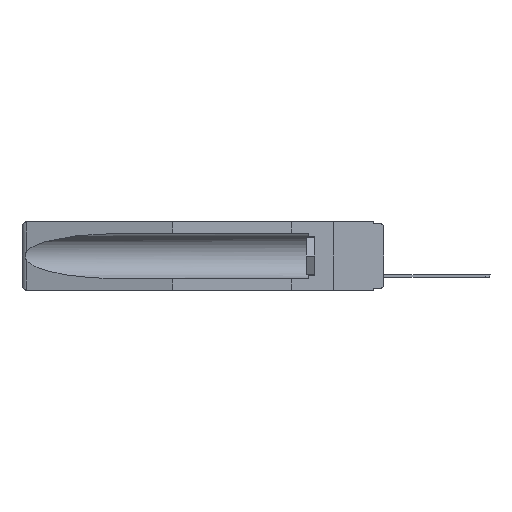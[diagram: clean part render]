
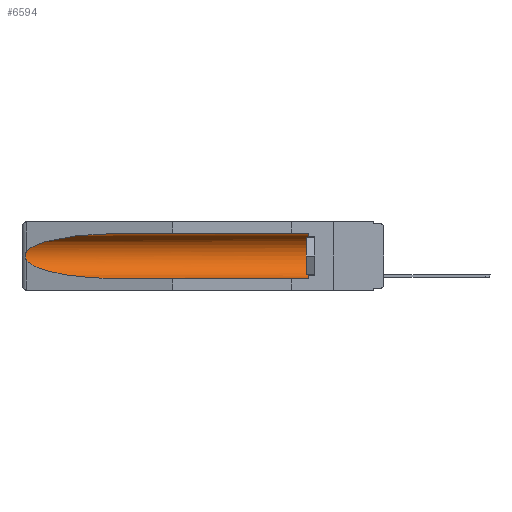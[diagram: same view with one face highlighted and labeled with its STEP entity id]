
A CAD part, left-side view. The second image highlights one B-rep face of the part: STEP entity #6594.
In plain terms, the highlighted cylindrical face has radius 2.857 mm (diameter 5.715 mm), a partial arc.
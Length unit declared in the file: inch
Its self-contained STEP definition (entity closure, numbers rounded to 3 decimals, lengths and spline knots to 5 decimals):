
#85 = VERTEX_POINT ( 'NONE', #4354 ) ;
#1199 = B_SPLINE_CURVE_WITH_KNOTS ( 'NONE', 3,
 ( #7776, #9515, #6013, #18506, #2538, #16663, #20144, #16814, #13372, #14959 ),
 .UNSPECIFIED., .F., .F.,
 ( 4, 2, 2, 2, 4 ),
 ( 0., 0.00029, 0.00058, 0.00087, 0.00117 ),
 .UNSPECIFIED. ) ;
#2200 = EDGE_CURVE ( 'NONE', #6729, #21876, #15597, .T. ) ;
#2538 = CARTESIAN_POINT ( 'NONE',  ( 0.2675, 1.53308, -0.16763 ) ) ;
#2858 = LINE ( 'NONE', #11179, #13998 ) ;
#3356 = CARTESIAN_POINT ( 'NONE',  ( 0.155, -0.30754, -0.1715 ) ) ;
#3700 = CARTESIAN_POINT ( 'NONE',  ( 0.155, -0.30754, -0.284 ) ) ;
#4354 = CARTESIAN_POINT ( 'NONE',  ( 0.26537, 1.52718, -0.19328 ) ) ;
#4469 = EDGE_CURVE ( 'NONE', #12045, #16624, #10929, .T. ) ;
#4706 = CARTESIAN_POINT ( 'NONE',  ( 0.21114, 1.30732, -0.284 ) ) ;
#5312 = CARTESIAN_POINT ( 'NONE',  ( 0.155, 0.126, -0.059 ) ) ;
#5488 = CARTESIAN_POINT ( 'NONE',  ( 0.155, 1.07973, -0.059 ) ) ;
#6013 = CARTESIAN_POINT ( 'NONE',  ( 0.26654, 1.53092, -0.15636 ) ) ;
#6271 = CARTESIAN_POINT ( 'NONE',  ( 0.26537, 1.52718, -0.19328 ) ) ;
#6594 = ADVANCED_FACE ( 'NONE', ( #17365 ), #7148, .F. ) ;
#6729 = VERTEX_POINT ( 'NONE', #5488 ) ;
#6937 = ORIENTED_EDGE ( 'NONE', *, *, #21263, .T. ) ;
#7148 = CYLINDRICAL_SURFACE ( 'NONE', #17399, 0.1125 ) ;
#7776 = CARTESIAN_POINT ( 'NONE',  ( 0.26537, 1.52718, -0.14972 ) ) ;
#8083 = CARTESIAN_POINT ( 'NONE',  ( 0.25451, 1.48313, -0.09465 ) ) ;
#9476 = VERTEX_POINT ( 'NONE', #20784 ) ;
#9515 = CARTESIAN_POINT ( 'NONE',  ( 0.26597, 1.52961, -0.15275 ) ) ;
#9613 = DIRECTION ( 'NONE',  ( 0., 0., 1. ) ) ;
#10467 = DIRECTION ( 'NONE',  ( 0., 1., 0. ) ) ;
#10908 = ORIENTED_EDGE ( 'NONE', *, *, #2200, .T. ) ;
#10929 = CIRCLE ( 'NONE', #20479, 0.1125 ) ;
#11139 = ORIENTED_EDGE ( 'NONE', *, *, #4469, .T. ) ;
#11179 = CARTESIAN_POINT ( 'NONE',  ( 0.155, -0.30754, -0.059 ) ) ;
#11735 = CARTESIAN_POINT ( 'NONE',  ( 0.26537, 1.52718, -0.14972 ) ) ;
#11904 =( BOUNDED_CURVE ( )  B_SPLINE_CURVE ( 3, ( #6271, #22373, #4706, #17071 ),
 .UNSPECIFIED., .F., .F. ) 
 B_SPLINE_CURVE_WITH_KNOTS ( ( 4, 4 ),
 ( 0.1948, 1.5708 ),
 .UNSPECIFIED. ) 
 CURVE ( )  GEOMETRIC_REPRESENTATION_ITEM ( )  RATIONAL_B_SPLINE_CURVE ( ( 1., 0.848, 0.848, 1. ) ) 
 REPRESENTATION_ITEM ( '' )  );
#11926 = ORIENTED_EDGE ( 'NONE', *, *, #13348, .T. ) ;
#12045 = VERTEX_POINT ( 'NONE', #14932 ) ;
#12816 = EDGE_LOOP ( 'NONE', ( #10908, #6937, #11926, #21684, #11139, #21150 ) ) ;
#13153 = LINE ( 'NONE', #3700, #19190 ) ;
#13348 = EDGE_CURVE ( 'NONE', #85, #9476, #11904, .T. ) ;
#13372 = CARTESIAN_POINT ( 'NONE',  ( 0.26597, 1.5296, -0.19026 ) ) ;
#13998 = VECTOR ( 'NONE', #18310, 39.37008 ) ;
#14932 = CARTESIAN_POINT ( 'NONE',  ( 0.155, 0.126, -0.284 ) ) ;
#14959 = CARTESIAN_POINT ( 'NONE',  ( 0.26537, 1.52718, -0.19328 ) ) ;
#15597 =( BOUNDED_CURVE ( )  B_SPLINE_CURVE ( 3, ( #19995, #19843, #8083, #11735 ),
 .UNSPECIFIED., .F., .F. ) 
 B_SPLINE_CURVE_WITH_KNOTS ( ( 4, 4 ),
 ( 4.71239, 6.08839 ),
 .UNSPECIFIED. ) 
 CURVE ( )  GEOMETRIC_REPRESENTATION_ITEM ( )  RATIONAL_B_SPLINE_CURVE ( ( 1., 0.848, 0.848, 1. ) ) 
 REPRESENTATION_ITEM ( '' )  );
#16566 = CARTESIAN_POINT ( 'NONE',  ( 0.26537, 1.52718, -0.14972 ) ) ;
#16624 = VERTEX_POINT ( 'NONE', #5312 ) ;
#16663 = CARTESIAN_POINT ( 'NONE',  ( 0.2675, 1.53308, -0.17534 ) ) ;
#16814 = CARTESIAN_POINT ( 'NONE',  ( 0.26655, 1.53094, -0.18657 ) ) ;
#17071 = CARTESIAN_POINT ( 'NONE',  ( 0.155, 1.07973, -0.284 ) ) ;
#17365 = FACE_OUTER_BOUND ( 'NONE', #12816, .T. ) ;
#17399 = AXIS2_PLACEMENT_3D ( 'NONE', #3356, #10467, #22836 ) ;
#17442 = EDGE_CURVE ( 'NONE', #16624, #6729, #2858, .T. ) ;
#18158 = CARTESIAN_POINT ( 'NONE',  ( 0.155, 0.126, -0.1715 ) ) ;
#18230 = DIRECTION ( 'NONE',  ( 0., -1., 0. ) ) ;
#18310 = DIRECTION ( 'NONE',  ( 0., 1., 0. ) ) ;
#18506 = CARTESIAN_POINT ( 'NONE',  ( 0.2673, 1.5327, -0.16383 ) ) ;
#18692 = EDGE_CURVE ( 'NONE', #12045, #9476, #13153, .T. ) ;
#19190 = VECTOR ( 'NONE', #19495, 39.37008 ) ;
#19495 = DIRECTION ( 'NONE',  ( 0., 1., 0. ) ) ;
#19843 = CARTESIAN_POINT ( 'NONE',  ( 0.21114, 1.30732, -0.059 ) ) ;
#19995 = CARTESIAN_POINT ( 'NONE',  ( 0.155, 1.07973, -0.059 ) ) ;
#20144 = CARTESIAN_POINT ( 'NONE',  ( 0.2673, 1.53269, -0.17917 ) ) ;
#20479 = AXIS2_PLACEMENT_3D ( 'NONE', #18158, #18230, #9613 ) ;
#20784 = CARTESIAN_POINT ( 'NONE',  ( 0.155, 1.07973, -0.284 ) ) ;
#21150 = ORIENTED_EDGE ( 'NONE', *, *, #17442, .T. ) ;
#21263 = EDGE_CURVE ( 'NONE', #21876, #85, #1199, .T. ) ;
#21684 = ORIENTED_EDGE ( 'NONE', *, *, #18692, .F. ) ;
#21876 = VERTEX_POINT ( 'NONE', #16566 ) ;
#22373 = CARTESIAN_POINT ( 'NONE',  ( 0.25451, 1.48313, -0.24835 ) ) ;
#22836 = DIRECTION ( 'NONE',  ( 0., 0., 1. ) ) ;
